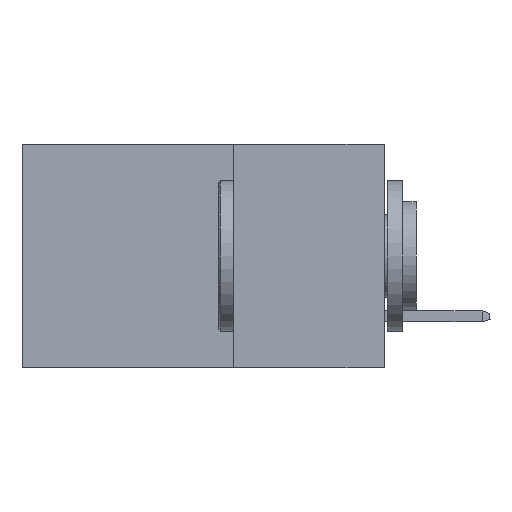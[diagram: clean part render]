
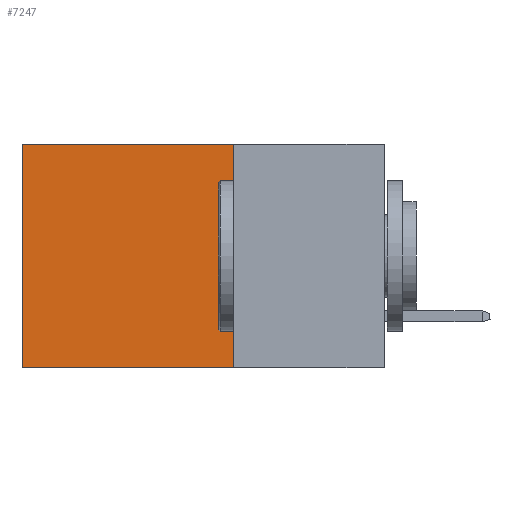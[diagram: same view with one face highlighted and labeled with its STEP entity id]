
A CAD part, left-side view. The second image highlights one B-rep face of the part: STEP entity #7247.
In plain terms, the highlighted planar face has unit normal (-1, 0, 0).
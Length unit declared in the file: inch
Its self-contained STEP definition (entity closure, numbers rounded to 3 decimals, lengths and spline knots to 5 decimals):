
#343 = CARTESIAN_POINT ( 'NONE',  ( 0.298, 0.25, 0. ) ) ;
#832 = VERTEX_POINT ( 'NONE', #15288 ) ;
#3709 = ORIENTED_EDGE ( 'NONE', *, *, #9533, .T. ) ;
#4956 = AXIS2_PLACEMENT_3D ( 'NONE', #343, #21378, #7436 ) ;
#5126 = PLANE ( 'NONE',  #4956 ) ;
#6198 = CARTESIAN_POINT ( 'NONE',  ( 0.298, 0.25, 0. ) ) ;
#6517 = CARTESIAN_POINT ( 'NONE',  ( 0.298, 0.25, 0. ) ) ;
#6793 = LINE ( 'NONE', #14172, #12292 ) ;
#7247 = ADVANCED_FACE ( 'NONE', ( #26050 ), #5126, .F. ) ;
#7436 = DIRECTION ( 'NONE',  ( 0., 0., -1. ) ) ;
#8539 = DIRECTION ( 'NONE',  ( 0., 0., -1. ) ) ;
#9533 = EDGE_CURVE ( 'NONE', #832, #29343, #23754, .T. ) ;
#11029 = ORIENTED_EDGE ( 'NONE', *, *, #27267, .F. ) ;
#12292 = VECTOR ( 'NONE', #27965, 39.37008 ) ;
#12591 = DIRECTION ( 'NONE',  ( 0., 0., -1. ) ) ;
#13420 = ORIENTED_EDGE ( 'NONE', *, *, #28318, .T. ) ;
#14172 = CARTESIAN_POINT ( 'NONE',  ( 0.298, 0.25, -0.37 ) ) ;
#15288 = CARTESIAN_POINT ( 'NONE',  ( 0.298, 0.25, 0. ) ) ;
#19479 = CARTESIAN_POINT ( 'NONE',  ( 0.298, 0.6, 0. ) ) ;
#19512 = EDGE_CURVE ( 'NONE', #24932, #27270, #6793, .T. ) ;
#20833 = VECTOR ( 'NONE', #12591, 39.37008 ) ;
#21378 = DIRECTION ( 'NONE',  ( 1., 0., 0. ) ) ;
#22465 = CARTESIAN_POINT ( 'NONE',  ( 0.298, 0.6, -0.37 ) ) ;
#22716 = LINE ( 'NONE', #6198, #28797 ) ;
#23021 = VECTOR ( 'NONE', #29671, 39.37008 ) ;
#23754 = LINE ( 'NONE', #6517, #23021 ) ;
#24932 = VERTEX_POINT ( 'NONE', #28942 ) ;
#26050 = FACE_OUTER_BOUND ( 'NONE', #29445, .T. ) ;
#26943 = LINE ( 'NONE', #19479, #20833 ) ;
#27267 = EDGE_CURVE ( 'NONE', #832, #24932, #22716, .T. ) ;
#27270 = VERTEX_POINT ( 'NONE', #22465 ) ;
#27402 = CARTESIAN_POINT ( 'NONE',  ( 0.298, 0.6, 0. ) ) ;
#27965 = DIRECTION ( 'NONE',  ( 0., 1., 0. ) ) ;
#28318 = EDGE_CURVE ( 'NONE', #29343, #27270, #26943, .T. ) ;
#28797 = VECTOR ( 'NONE', #8539, 39.37008 ) ;
#28942 = CARTESIAN_POINT ( 'NONE',  ( 0.298, 0.25, -0.37 ) ) ;
#29343 = VERTEX_POINT ( 'NONE', #27402 ) ;
#29445 = EDGE_LOOP ( 'NONE', ( #13420, #29616, #11029, #3709 ) ) ;
#29616 = ORIENTED_EDGE ( 'NONE', *, *, #19512, .F. ) ;
#29671 = DIRECTION ( 'NONE',  ( 0., 1., 0. ) ) ;
